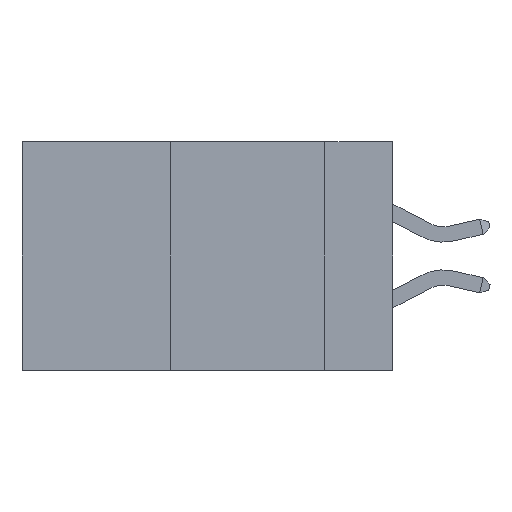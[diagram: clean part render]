
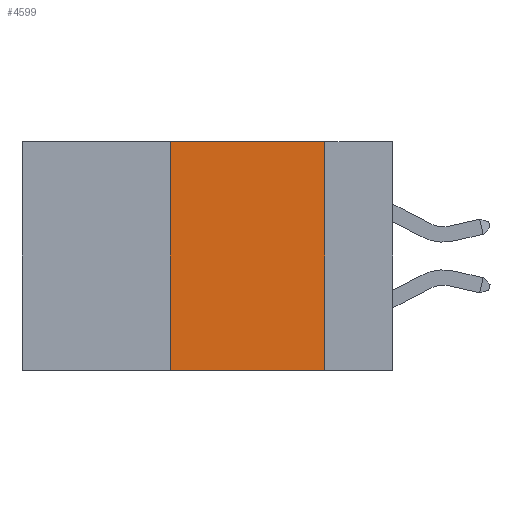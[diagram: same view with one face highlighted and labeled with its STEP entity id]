
A CAD part, left-side view. The second image highlights one B-rep face of the part: STEP entity #4599.
In plain terms, the highlighted planar face has unit normal (-1, 0, 0).
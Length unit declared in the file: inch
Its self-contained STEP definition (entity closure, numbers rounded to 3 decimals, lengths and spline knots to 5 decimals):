
#49 = ORIENTED_EDGE ( 'NONE', *, *, #2194, .T. ) ;
#914 = LINE ( 'NONE', #9104, #16071 ) ;
#2194 = EDGE_CURVE ( 'NONE', #3328, #18395, #17875, .T. ) ;
#3328 = VERTEX_POINT ( 'NONE', #13508 ) ;
#4396 = CARTESIAN_POINT ( 'NONE',  ( 0., 0.6, 0. ) ) ;
#4599 = ADVANCED_FACE ( 'NONE', ( #17300 ), #13252, .F. ) ;
#5939 = CARTESIAN_POINT ( 'NONE',  ( 0., 0.6, 0. ) ) ;
#6427 = VECTOR ( 'NONE', #15857, 39.37008 ) ;
#6581 = EDGE_CURVE ( 'NONE', #10600, #18395, #17953, .T. ) ;
#8571 = ORIENTED_EDGE ( 'NONE', *, *, #6581, .F. ) ;
#9047 = ORIENTED_EDGE ( 'NONE', *, *, #16173, .F. ) ;
#9104 = CARTESIAN_POINT ( 'NONE',  ( 0., 0.36, 0. ) ) ;
#10055 = AXIS2_PLACEMENT_3D ( 'NONE', #4396, #14728, #11639 ) ;
#10163 = VERTEX_POINT ( 'NONE', #11931 ) ;
#10168 = CARTESIAN_POINT ( 'NONE',  ( 0., 0.11, 0. ) ) ;
#10412 = CARTESIAN_POINT ( 'NONE',  ( 0., 0.11, 0. ) ) ;
#10600 = VERTEX_POINT ( 'NONE', #10412 ) ;
#11228 = EDGE_CURVE ( 'NONE', #10163, #10600, #18717, .T. ) ;
#11639 = DIRECTION ( 'NONE',  ( 0., 0., -1. ) ) ;
#11931 = CARTESIAN_POINT ( 'NONE',  ( 0., 0.36, 0. ) ) ;
#11937 = DIRECTION ( 'NONE',  ( 0., -1., 0. ) ) ;
#12053 = DIRECTION ( 'NONE',  ( 0., 0., 1. ) ) ;
#12178 = CARTESIAN_POINT ( 'NONE',  ( 0., 0.11, -0.37 ) ) ;
#13104 = EDGE_LOOP ( 'NONE', ( #8571, #16994, #9047, #49 ) ) ;
#13252 = PLANE ( 'NONE',  #10055 ) ;
#13508 = CARTESIAN_POINT ( 'NONE',  ( 0., 0.36, -0.37 ) ) ;
#14125 = VECTOR ( 'NONE', #17484, 39.37008 ) ;
#14423 = CARTESIAN_POINT ( 'NONE',  ( 0., 0.6, -0.37 ) ) ;
#14728 = DIRECTION ( 'NONE',  ( 1., 0., 0. ) ) ;
#15857 = DIRECTION ( 'NONE',  ( 0., -1., 0. ) ) ;
#16071 = VECTOR ( 'NONE', #12053, 39.37008 ) ;
#16173 = EDGE_CURVE ( 'NONE', #3328, #10163, #914, .T. ) ;
#16994 = ORIENTED_EDGE ( 'NONE', *, *, #11228, .F. ) ;
#17300 = FACE_OUTER_BOUND ( 'NONE', #13104, .T. ) ;
#17484 = DIRECTION ( 'NONE',  ( 0., 0., -1. ) ) ;
#17875 = LINE ( 'NONE', #14423, #6427 ) ;
#17953 = LINE ( 'NONE', #10168, #14125 ) ;
#18395 = VERTEX_POINT ( 'NONE', #12178 ) ;
#18501 = VECTOR ( 'NONE', #11937, 39.37008 ) ;
#18717 = LINE ( 'NONE', #5939, #18501 ) ;
